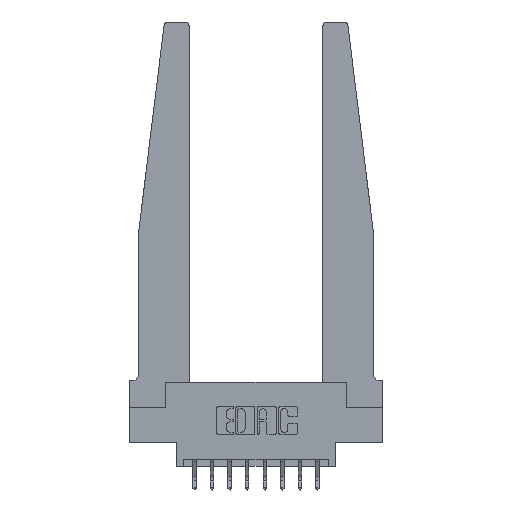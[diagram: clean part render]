
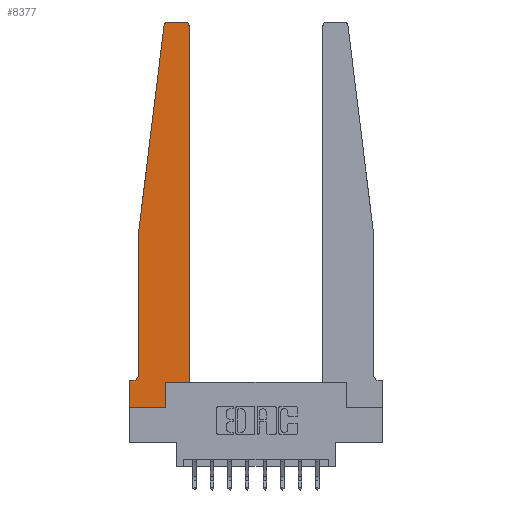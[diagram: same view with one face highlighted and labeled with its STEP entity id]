
A CAD part, top view. The second image highlights one B-rep face of the part: STEP entity #8377.
In plain terms, the highlighted planar face has unit normal (0, 0, 1).
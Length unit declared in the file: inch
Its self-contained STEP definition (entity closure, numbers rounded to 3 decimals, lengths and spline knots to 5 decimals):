
#112 = ORIENTED_EDGE ( 'NONE', *, *, #11697, .T. ) ;
#475 = LINE ( 'NONE', #7492, #557 ) ;
#557 = VECTOR ( 'NONE', #3741, 39.37008 ) ;
#598 = VERTEX_POINT ( 'NONE', #10796 ) ;
#1080 = CARTESIAN_POINT ( 'NONE',  ( 0.2605, 0.18, 0.37 ) ) ;
#1167 = VERTEX_POINT ( 'NONE', #3040 ) ;
#1232 = CARTESIAN_POINT ( 'NONE',  ( 0., 0., 0.37 ) ) ;
#1251 = ORIENTED_EDGE ( 'NONE', *, *, #9586, .T. ) ;
#1289 = VERTEX_POINT ( 'NONE', #1080 ) ;
#1338 = VERTEX_POINT ( 'NONE', #10615 ) ;
#1388 = CARTESIAN_POINT ( 'NONE',  ( 0.065, 0.2375, 0.37 ) ) ;
#1420 = CARTESIAN_POINT ( 'NONE',  ( 0.395, 2.72, 0.37 ) ) ;
#1748 = CARTESIAN_POINT ( 'NONE',  ( 0., 0., 0.37 ) ) ;
#1764 = DIRECTION ( 'NONE',  ( 0., -1., 0. ) ) ;
#1785 = ORIENTED_EDGE ( 'NONE', *, *, #14242, .T. ) ;
#1860 = EDGE_LOOP ( 'NONE', ( #13846, #4114, #8110, #14786, #112, #1251, #15115, #15187, #1785, #11629, #5021, #12974 ) ) ;
#1952 = EDGE_CURVE ( 'NONE', #11300, #13107, #8445, .T. ) ;
#1990 = EDGE_CURVE ( 'NONE', #13107, #12892, #2686, .T. ) ;
#2126 = PLANE ( 'NONE',  #8538 ) ;
#2195 = CARTESIAN_POINT ( 'NONE',  ( 0.065, 1.25, 0.37 ) ) ;
#2257 = DIRECTION ( 'NONE',  ( -1., 0., 0. ) ) ;
#2582 = CARTESIAN_POINT ( 'NONE',  ( 0., 0.1875, 0.37 ) ) ;
#2593 = VECTOR ( 'NONE', #8398, 39.37008 ) ;
#2661 = DIRECTION ( 'NONE',  ( 0., 0., 1. ) ) ;
#2686 = LINE ( 'NONE', #1748, #14784 ) ;
#2780 = LINE ( 'NONE', #6274, #6528 ) ;
#3040 = CARTESIAN_POINT ( 'NONE',  ( 0.425, 2.72, 0.37 ) ) ;
#3528 = LINE ( 'NONE', #5875, #11943 ) ;
#3640 = VERTEX_POINT ( 'NONE', #8114 ) ;
#3741 = DIRECTION ( 'NONE',  ( -1., 0., 0. ) ) ;
#3800 = CIRCLE ( 'NONE', #13497, 0.03 ) ;
#4071 = VECTOR ( 'NONE', #12162, 39.37008 ) ;
#4107 = DIRECTION ( 'NONE',  ( -1., 0., 0. ) ) ;
#4114 = ORIENTED_EDGE ( 'NONE', *, *, #8270, .T. ) ;
#4205 = DIRECTION ( 'NONE',  ( 1., 0., 0. ) ) ;
#4334 = DIRECTION ( 'NONE',  ( 0., 0., -1. ) ) ;
#4352 = DIRECTION ( 'NONE',  ( 0., 0., 1. ) ) ;
#4901 = CARTESIAN_POINT ( 'NONE',  ( 0.065, 1.25, 0.37 ) ) ;
#4939 = LINE ( 'NONE', #9667, #4071 ) ;
#5021 = ORIENTED_EDGE ( 'NONE', *, *, #9501, .T. ) ;
#5265 = CARTESIAN_POINT ( 'NONE',  ( 0.015, 0.2375, 0.37 ) ) ;
#5324 = EDGE_CURVE ( 'NONE', #1167, #13700, #3800, .T. ) ;
#5617 = CARTESIAN_POINT ( 'NONE',  ( 0.2605, 0.18, 0.37 ) ) ;
#5875 = CARTESIAN_POINT ( 'NONE',  ( 0.425, 0.18, 0.37 ) ) ;
#6052 = CIRCLE ( 'NONE', #10979, 0.03 ) ;
#6274 = CARTESIAN_POINT ( 'NONE',  ( 0.065, 1.25, 0.37 ) ) ;
#6467 = CARTESIAN_POINT ( 'NONE',  ( 0.2605, 0., 0.37 ) ) ;
#6528 = VECTOR ( 'NONE', #1764, 39.37008 ) ;
#7078 = CIRCLE ( 'NONE', #9055, 0.05 ) ;
#7198 = EDGE_CURVE ( 'NONE', #13700, #3640, #10537, .T. ) ;
#7492 = CARTESIAN_POINT ( 'NONE',  ( 0.065, 0.1875, 0.37 ) ) ;
#8110 = ORIENTED_EDGE ( 'NONE', *, *, #9688, .T. ) ;
#8114 = CARTESIAN_POINT ( 'NONE',  ( 0.27653, 2.75, 0.37 ) ) ;
#8270 = EDGE_CURVE ( 'NONE', #3640, #1338, #6052, .T. ) ;
#8332 = CARTESIAN_POINT ( 'NONE',  ( 0.015, 0.1875, 0.37 ) ) ;
#8352 = DIRECTION ( 'NONE',  ( 1., 0., 0. ) ) ;
#8377 = ADVANCED_FACE ( 'NONE', ( #10412 ), #2126, .T. ) ;
#8398 = DIRECTION ( 'NONE',  ( 0., 1., 0. ) ) ;
#8445 = LINE ( 'NONE', #10735, #14429 ) ;
#8538 = AXIS2_PLACEMENT_3D ( 'NONE', #12588, #4352, #13761 ) ;
#8878 = CARTESIAN_POINT ( 'NONE',  ( 0.27653, 2.72, 0.37 ) ) ;
#8885 = EDGE_CURVE ( 'NONE', #11261, #13304, #2780, .T. ) ;
#9055 = AXIS2_PLACEMENT_3D ( 'NONE', #5265, #4334, #4107 ) ;
#9501 = EDGE_CURVE ( 'NONE', #598, #1167, #3528, .T. ) ;
#9586 = EDGE_CURVE ( 'NONE', #15110, #11300, #475, .T. ) ;
#9667 = CARTESIAN_POINT ( 'NONE',  ( 0.425, 0.18, 0.37 ) ) ;
#9688 = EDGE_CURVE ( 'NONE', #1338, #11261, #14063, .T. ) ;
#9815 = DIRECTION ( 'NONE',  ( 1., 0., 0. ) ) ;
#10412 = FACE_OUTER_BOUND ( 'NONE', #1860, .T. ) ;
#10499 = DIRECTION ( 'NONE',  ( 0., 1., 0. ) ) ;
#10537 = LINE ( 'NONE', #11541, #13967 ) ;
#10599 = DIRECTION ( 'NONE',  ( 0., -1., 0. ) ) ;
#10615 = CARTESIAN_POINT ( 'NONE',  ( 0.24675, 2.72367, 0.37 ) ) ;
#10735 = CARTESIAN_POINT ( 'NONE',  ( 0., 0., 0.37 ) ) ;
#10796 = CARTESIAN_POINT ( 'NONE',  ( 0.425, 0.18, 0.37 ) ) ;
#10979 = AXIS2_PLACEMENT_3D ( 'NONE', #8878, #13609, #4205 ) ;
#11261 = VERTEX_POINT ( 'NONE', #4901 ) ;
#11300 = VERTEX_POINT ( 'NONE', #2582 ) ;
#11541 = CARTESIAN_POINT ( 'NONE',  ( 0.25, 2.75, 0.37 ) ) ;
#11629 = ORIENTED_EDGE ( 'NONE', *, *, #14357, .T. ) ;
#11645 = LINE ( 'NONE', #5617, #2593 ) ;
#11697 = EDGE_CURVE ( 'NONE', #13304, #15110, #7078, .T. ) ;
#11943 = VECTOR ( 'NONE', #10499, 39.37008 ) ;
#12162 = DIRECTION ( 'NONE',  ( 1., 0., 0. ) ) ;
#12588 = CARTESIAN_POINT ( 'NONE',  ( 0., 0.1875, 0.37 ) ) ;
#12710 = VECTOR ( 'NONE', #14779, 39.37008 ) ;
#12892 = VERTEX_POINT ( 'NONE', #6467 ) ;
#12974 = ORIENTED_EDGE ( 'NONE', *, *, #5324, .T. ) ;
#13107 = VERTEX_POINT ( 'NONE', #1232 ) ;
#13304 = VERTEX_POINT ( 'NONE', #1388 ) ;
#13497 = AXIS2_PLACEMENT_3D ( 'NONE', #1420, #2661, #8352 ) ;
#13609 = DIRECTION ( 'NONE',  ( 0., 0., 1. ) ) ;
#13700 = VERTEX_POINT ( 'NONE', #13782 ) ;
#13761 = DIRECTION ( 'NONE',  ( 1., 0., 0. ) ) ;
#13782 = CARTESIAN_POINT ( 'NONE',  ( 0.395, 2.75, 0.37 ) ) ;
#13846 = ORIENTED_EDGE ( 'NONE', *, *, #7198, .T. ) ;
#13967 = VECTOR ( 'NONE', #2257, 39.37008 ) ;
#14063 = LINE ( 'NONE', #2195, #12710 ) ;
#14242 = EDGE_CURVE ( 'NONE', #12892, #1289, #11645, .T. ) ;
#14357 = EDGE_CURVE ( 'NONE', #1289, #598, #4939, .T. ) ;
#14429 = VECTOR ( 'NONE', #10599, 39.37008 ) ;
#14779 = DIRECTION ( 'NONE',  ( -0.122, -0.992, 0. ) ) ;
#14784 = VECTOR ( 'NONE', #9815, 39.37008 ) ;
#14786 = ORIENTED_EDGE ( 'NONE', *, *, #8885, .T. ) ;
#15110 = VERTEX_POINT ( 'NONE', #8332 ) ;
#15115 = ORIENTED_EDGE ( 'NONE', *, *, #1952, .T. ) ;
#15187 = ORIENTED_EDGE ( 'NONE', *, *, #1990, .T. ) ;
